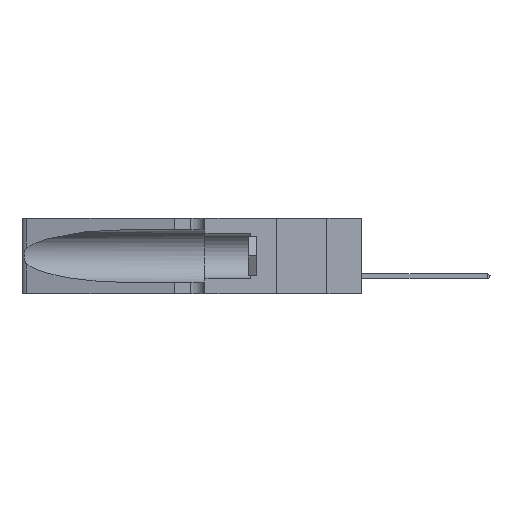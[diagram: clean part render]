
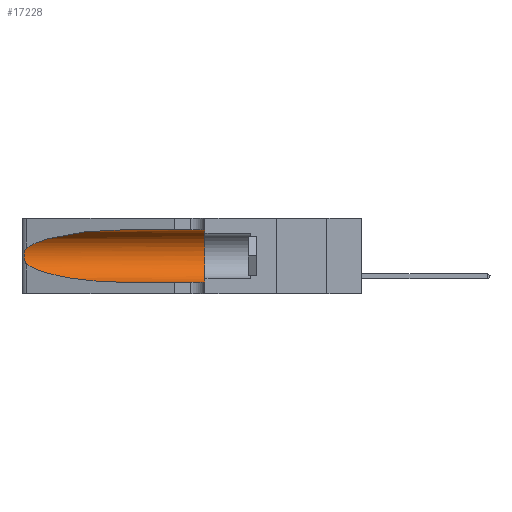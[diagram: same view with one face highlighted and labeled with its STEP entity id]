
A CAD part, left-side view. The second image highlights one B-rep face of the part: STEP entity #17228.
In plain terms, the highlighted cylindrical face has radius 3.308 mm (diameter 6.617 mm), a partial arc.
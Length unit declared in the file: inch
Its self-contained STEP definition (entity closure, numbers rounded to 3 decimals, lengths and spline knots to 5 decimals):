
#866 = VERTEX_POINT ( 'NONE', #18934 ) ;
#1939 = CARTESIAN_POINT ( 'NONE',  ( 0.25487, 1.22718, 0.22369 ) ) ;
#2056 = CARTESIAN_POINT ( 'NONE',  ( 0.18966, 0.96281, 0.05475 ) ) ;
#2432 = B_SPLINE_CURVE_WITH_KNOTS ( 'NONE', 3,
 ( #28891, #3912, #19184, #28372, #35130, #28759, #34734, #37884, #16568, #28498, #13197, #38264, #9966, #19460 ),
 .UNSPECIFIED., .F., .F.,
 ( 4, 2, 2, 2, 2, 2, 4 ),
 ( 0., 0.00027, 0.00053, 0.00107, 0.0016, 0.00187, 0.00214 ),
 .UNSPECIFIED. ) ;
#2620 = CARTESIAN_POINT ( 'NONE',  ( 0.1305, 1.61858, 0.31525 ) ) ;
#3280 = EDGE_LOOP ( 'NONE', ( #5467, #35193, #13388, #31256, #39612, #10395 ) ) ;
#3396 = CARTESIAN_POINT ( 'NONE',  ( 0.1305, 0.72297, 0.31525 ) ) ;
#3912 = CARTESIAN_POINT ( 'NONE',  ( 0.25555, 1.22994, 0.2215 ) ) ;
#4524 = VERTEX_POINT ( 'NONE', #1939 ) ;
#5467 = ORIENTED_EDGE ( 'NONE', *, *, #33463, .T. ) ;
#5581 = DIRECTION ( 'NONE',  ( 0., -1., 0. ) ) ;
#6352 = CARTESIAN_POINT ( 'NONE',  ( 0.2373, 1.15595, 0.28018 ) ) ;
#7739 = CARTESIAN_POINT ( 'NONE',  ( 0.1305, 1.61858, 0.185 ) ) ;
#7817 = EDGE_CURVE ( 'NONE', #13292, #866, #21428, .T. ) ;
#8636 = DIRECTION ( 'NONE',  ( 0., 1., 0. ) ) ;
#9119 = EDGE_CURVE ( 'NONE', #23266, #36570, #12567, .T. ) ;
#9708 = FACE_OUTER_BOUND ( 'NONE', #3280, .T. ) ;
#9756 = CARTESIAN_POINT ( 'NONE',  ( 0.25487, 1.22718, 0.14631 ) ) ;
#9966 = CARTESIAN_POINT ( 'NONE',  ( 0.25555, 1.22993, 0.14849 ) ) ;
#10395 = ORIENTED_EDGE ( 'NONE', *, *, #28010, .F. ) ;
#11348 = CARTESIAN_POINT ( 'NONE',  ( 0.1305, 0.72297, 0.05475 ) ) ;
#11471 = CARTESIAN_POINT ( 'NONE',  ( 0.25487, 1.22718, 0.14631 ) ) ;
#11649 = LINE ( 'NONE', #2620, #20873 ) ;
#12567 =( BOUNDED_CURVE ( )  B_SPLINE_CURVE ( 3, ( #11471, #23297, #2056, #11348 ),
 .UNSPECIFIED., .F., .F. ) 
 B_SPLINE_CURVE_WITH_KNOTS ( ( 4, 4 ),
 ( 3.44316, 4.71239 ),
 .UNSPECIFIED. ) 
 CURVE ( )  GEOMETRIC_REPRESENTATION_ITEM ( )  RATIONAL_B_SPLINE_CURVE ( ( 1., 0.87, 0.87, 1. ) ) 
 REPRESENTATION_ITEM ( '' )  );
#12892 = EDGE_CURVE ( 'NONE', #4524, #23266, #2432, .T. ) ;
#13197 = CARTESIAN_POINT ( 'NONE',  ( 0.25789, 1.23486, 0.15765 ) ) ;
#13292 = VERTEX_POINT ( 'NONE', #30624 ) ;
#13388 = ORIENTED_EDGE ( 'NONE', *, *, #9119, .T. ) ;
#14274 = DIRECTION ( 'NONE',  ( 0., 0., 1. ) ) ;
#16568 = CARTESIAN_POINT ( 'NONE',  ( 0.26017, 1.23833, 0.17102 ) ) ;
#17228 = ADVANCED_FACE ( 'NONE', ( #9708 ), #25659, .F. ) ;
#18536 = DIRECTION ( 'NONE',  ( 0., 0., -1. ) ) ;
#18789 = CARTESIAN_POINT ( 'NONE',  ( 0.18966, 0.96281, 0.31525 ) ) ;
#18934 = CARTESIAN_POINT ( 'NONE',  ( 0.1305, 0.35, 0.05475 ) ) ;
#19133 = EDGE_CURVE ( 'NONE', #36570, #866, #39635, .T. ) ;
#19184 = CARTESIAN_POINT ( 'NONE',  ( 0.25639, 1.23184, 0.21858 ) ) ;
#19460 = CARTESIAN_POINT ( 'NONE',  ( 0.25487, 1.22718, 0.14631 ) ) ;
#20873 = VECTOR ( 'NONE', #33420, 39.37008 ) ;
#21428 = CIRCLE ( 'NONE', #34090, 0.13025 ) ;
#23088 = VERTEX_POINT ( 'NONE', #36472 ) ;
#23266 = VERTEX_POINT ( 'NONE', #9756 ) ;
#23297 = CARTESIAN_POINT ( 'NONE',  ( 0.2373, 1.15595, 0.08982 ) ) ;
#23728 = DIRECTION ( 'NONE',  ( 0., -1., 0. ) ) ;
#24047 = CARTESIAN_POINT ( 'NONE',  ( 0.1305, 0.35, 0.185 ) ) ;
#25659 = CYLINDRICAL_SURFACE ( 'NONE', #26050, 0.13025 ) ;
#26050 = AXIS2_PLACEMENT_3D ( 'NONE', #7739, #5581, #18536 ) ;
#26826 = CARTESIAN_POINT ( 'NONE',  ( 0.1305, 1.61858, 0.05475 ) ) ;
#27718 = CARTESIAN_POINT ( 'NONE',  ( 0.25487, 1.22718, 0.22369 ) ) ;
#27998 = VECTOR ( 'NONE', #23728, 39.37008 ) ;
#28010 = EDGE_CURVE ( 'NONE', #23088, #13292, #11649, .T. ) ;
#28372 = CARTESIAN_POINT ( 'NONE',  ( 0.25787, 1.23484, 0.2124 ) ) ;
#28498 = CARTESIAN_POINT ( 'NONE',  ( 0.25856, 1.23593, 0.16098 ) ) ;
#28759 = CARTESIAN_POINT ( 'NONE',  ( 0.26018, 1.23835, 0.19895 ) ) ;
#28891 = CARTESIAN_POINT ( 'NONE',  ( 0.25487, 1.22718, 0.22369 ) ) ;
#29925 =( BOUNDED_CURVE ( )  B_SPLINE_CURVE ( 3, ( #3396, #18789, #6352, #27718 ),
 .UNSPECIFIED., .F., .F. ) 
 B_SPLINE_CURVE_WITH_KNOTS ( ( 4, 4 ),
 ( 1.5708, 2.84003 ),
 .UNSPECIFIED. ) 
 CURVE ( )  GEOMETRIC_REPRESENTATION_ITEM ( )  RATIONAL_B_SPLINE_CURVE ( ( 1., 0.87, 0.87, 1. ) ) 
 REPRESENTATION_ITEM ( '' )  );
#29974 = CARTESIAN_POINT ( 'NONE',  ( 0.1305, 0.72297, 0.05475 ) ) ;
#30624 = CARTESIAN_POINT ( 'NONE',  ( 0.1305, 0.35, 0.31525 ) ) ;
#31256 = ORIENTED_EDGE ( 'NONE', *, *, #19133, .T. ) ;
#33420 = DIRECTION ( 'NONE',  ( 0., -1., 0. ) ) ;
#33463 = EDGE_CURVE ( 'NONE', #23088, #4524, #29925, .T. ) ;
#34090 = AXIS2_PLACEMENT_3D ( 'NONE', #24047, #8636, #14274 ) ;
#34734 = CARTESIAN_POINT ( 'NONE',  ( 0.26075, 1.23896, 0.19203 ) ) ;
#35130 = CARTESIAN_POINT ( 'NONE',  ( 0.25854, 1.2359, 0.20912 ) ) ;
#35193 = ORIENTED_EDGE ( 'NONE', *, *, #12892, .T. ) ;
#36472 = CARTESIAN_POINT ( 'NONE',  ( 0.1305, 0.72297, 0.31525 ) ) ;
#36570 = VERTEX_POINT ( 'NONE', #29974 ) ;
#37884 = CARTESIAN_POINT ( 'NONE',  ( 0.26075, 1.23896, 0.178 ) ) ;
#38264 = CARTESIAN_POINT ( 'NONE',  ( 0.25639, 1.23186, 0.15144 ) ) ;
#39612 = ORIENTED_EDGE ( 'NONE', *, *, #7817, .F. ) ;
#39635 = LINE ( 'NONE', #26826, #27998 ) ;
